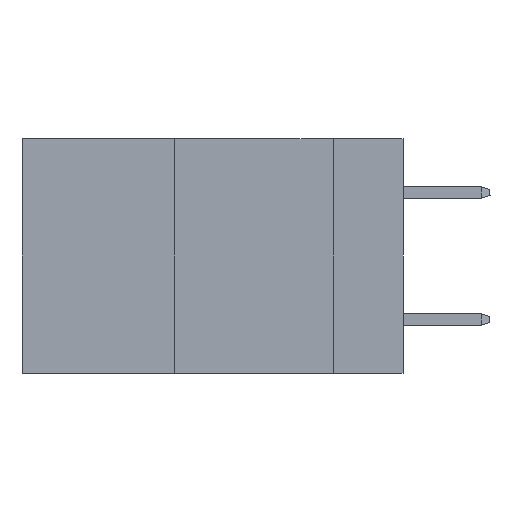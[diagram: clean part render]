
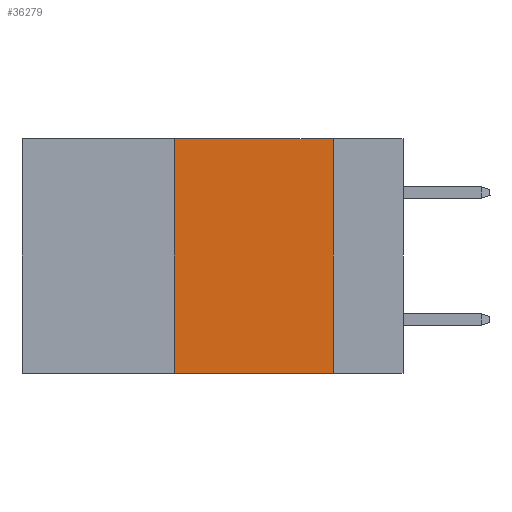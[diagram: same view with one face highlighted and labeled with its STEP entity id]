
A CAD part, left-side view. The second image highlights one B-rep face of the part: STEP entity #36279.
In plain terms, the highlighted planar face has unit normal (-1, 0, 0).
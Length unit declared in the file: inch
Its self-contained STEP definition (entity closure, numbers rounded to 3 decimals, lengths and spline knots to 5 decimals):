
#1081 = DIRECTION ( 'NONE',  ( 1., 0., 0. ) ) ;
#1309 = DIRECTION ( 'NONE',  ( 0., 0., -1. ) ) ;
#1392 = VECTOR ( 'NONE', #38021, 39.37008 ) ;
#1797 = CARTESIAN_POINT ( 'NONE',  ( 0., 0.6, -0.37 ) ) ;
#3150 = EDGE_CURVE ( 'NONE', #25235, #24907, #28834, .T. ) ;
#5366 = ORIENTED_EDGE ( 'NONE', *, *, #25085, .T. ) ;
#5879 = DIRECTION ( 'NONE',  ( 0., -1., 0. ) ) ;
#6404 = CARTESIAN_POINT ( 'NONE',  ( 0., 0.11, -0.37 ) ) ;
#8338 = EDGE_CURVE ( 'NONE', #44936, #43942, #37325, .T. ) ;
#10379 = CARTESIAN_POINT ( 'NONE',  ( 0., 0.36, 0. ) ) ;
#12916 = CARTESIAN_POINT ( 'NONE',  ( 0., 0.11, 0. ) ) ;
#17139 = VECTOR ( 'NONE', #39053, 39.37008 ) ;
#18173 = EDGE_LOOP ( 'NONE', ( #23926, #42226, #33262, #5366 ) ) ;
#22665 = PLANE ( 'NONE',  #23580 ) ;
#23580 = AXIS2_PLACEMENT_3D ( 'NONE', #37122, #1081, #1309 ) ;
#23926 = ORIENTED_EDGE ( 'NONE', *, *, #8338, .F. ) ;
#24907 = VERTEX_POINT ( 'NONE', #10379 ) ;
#25085 = EDGE_CURVE ( 'NONE', #25235, #43942, #26686, .T. ) ;
#25235 = VERTEX_POINT ( 'NONE', #45435 ) ;
#26215 = FACE_OUTER_BOUND ( 'NONE', #18173, .T. ) ;
#26686 = LINE ( 'NONE', #1797, #38135 ) ;
#28399 = LINE ( 'NONE', #45957, #45939 ) ;
#28834 = LINE ( 'NONE', #32373, #17139 ) ;
#30249 = DIRECTION ( 'NONE',  ( 0., -1., 0. ) ) ;
#32373 = CARTESIAN_POINT ( 'NONE',  ( 0., 0.36, 0. ) ) ;
#33262 = ORIENTED_EDGE ( 'NONE', *, *, #3150, .F. ) ;
#36279 = ADVANCED_FACE ( 'NONE', ( #26215 ), #22665, .F. ) ;
#37122 = CARTESIAN_POINT ( 'NONE',  ( 0., 0.6, 0. ) ) ;
#37325 = LINE ( 'NONE', #12916, #1392 ) ;
#38021 = DIRECTION ( 'NONE',  ( 0., 0., -1. ) ) ;
#38135 = VECTOR ( 'NONE', #30249, 39.37008 ) ;
#39053 = DIRECTION ( 'NONE',  ( 0., 0., 1. ) ) ;
#39961 = CARTESIAN_POINT ( 'NONE',  ( 0., 0.11, 0. ) ) ;
#42226 = ORIENTED_EDGE ( 'NONE', *, *, #44420, .F. ) ;
#43942 = VERTEX_POINT ( 'NONE', #6404 ) ;
#44420 = EDGE_CURVE ( 'NONE', #24907, #44936, #28399, .T. ) ;
#44936 = VERTEX_POINT ( 'NONE', #39961 ) ;
#45435 = CARTESIAN_POINT ( 'NONE',  ( 0., 0.36, -0.37 ) ) ;
#45939 = VECTOR ( 'NONE', #5879, 39.37008 ) ;
#45957 = CARTESIAN_POINT ( 'NONE',  ( 0., 0.6, 0. ) ) ;
